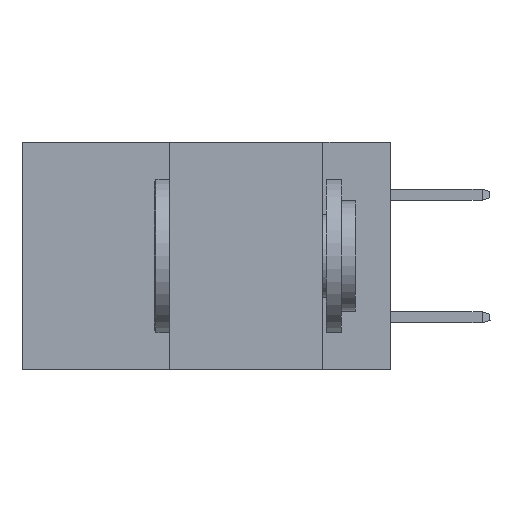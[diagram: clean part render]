
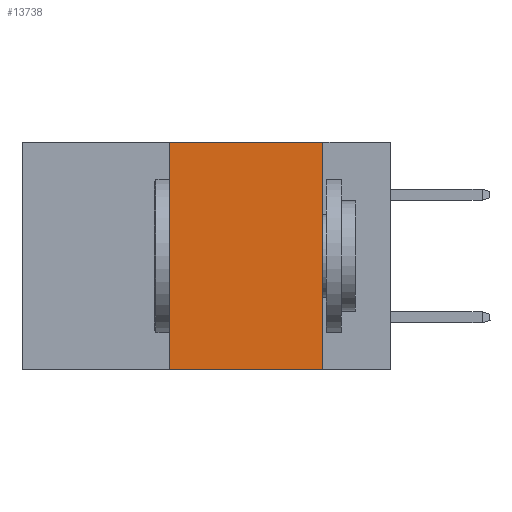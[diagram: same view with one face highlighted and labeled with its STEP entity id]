
A CAD part, left-side view. The second image highlights one B-rep face of the part: STEP entity #13738.
In plain terms, the highlighted planar face has unit normal (-1, 0, 0).
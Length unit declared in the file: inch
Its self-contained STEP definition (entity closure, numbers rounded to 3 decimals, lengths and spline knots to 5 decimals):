
#1080 = DIRECTION ( 'NONE',  ( 0., 0., 1. ) ) ;
#2075 = EDGE_CURVE ( 'NONE', #35773, #3460, #32425, .T. ) ;
#3299 = VERTEX_POINT ( 'NONE', #31021 ) ;
#3460 = VERTEX_POINT ( 'NONE', #13217 ) ;
#6713 = DIRECTION ( 'NONE',  ( 0., -1., 0. ) ) ;
#6886 = LINE ( 'NONE', #20181, #40118 ) ;
#6978 = VECTOR ( 'NONE', #37081, 39.37008 ) ;
#8865 = CARTESIAN_POINT ( 'NONE',  ( 0., 0.36, 0. ) ) ;
#10629 = VECTOR ( 'NONE', #36260, 39.37008 ) ;
#13023 = LINE ( 'NONE', #27232, #6978 ) ;
#13217 = CARTESIAN_POINT ( 'NONE',  ( 0., 0.11, -0.37 ) ) ;
#13467 = DIRECTION ( 'NONE',  ( 0., 0., -1. ) ) ;
#13738 = ADVANCED_FACE ( 'NONE', ( #32394 ), #39095, .F. ) ;
#18110 = EDGE_CURVE ( 'NONE', #3299, #3460, #38824, .T. ) ;
#18336 = VECTOR ( 'NONE', #6713, 39.37008 ) ;
#20181 = CARTESIAN_POINT ( 'NONE',  ( 0., 0.36, 0. ) ) ;
#21329 = ORIENTED_EDGE ( 'NONE', *, *, #34332, .F. ) ;
#26314 = ORIENTED_EDGE ( 'NONE', *, *, #2075, .T. ) ;
#26459 = DIRECTION ( 'NONE',  ( 1., 0., 0. ) ) ;
#26561 = CARTESIAN_POINT ( 'NONE',  ( 0., 0.11, 0. ) ) ;
#27232 = CARTESIAN_POINT ( 'NONE',  ( 0., 0.6, 0. ) ) ;
#28123 = ORIENTED_EDGE ( 'NONE', *, *, #36096, .F. ) ;
#29133 = EDGE_LOOP ( 'NONE', ( #31268, #21329, #28123, #26314 ) ) ;
#31021 = CARTESIAN_POINT ( 'NONE',  ( 0., 0.11, 0. ) ) ;
#31268 = ORIENTED_EDGE ( 'NONE', *, *, #18110, .F. ) ;
#31813 = CARTESIAN_POINT ( 'NONE',  ( 0., 0.6, -0.37 ) ) ;
#32303 = CARTESIAN_POINT ( 'NONE',  ( 0., 0.36, -0.37 ) ) ;
#32394 = FACE_OUTER_BOUND ( 'NONE', #29133, .T. ) ;
#32425 = LINE ( 'NONE', #31813, #18336 ) ;
#33072 = CARTESIAN_POINT ( 'NONE',  ( 0., 0.6, 0. ) ) ;
#34332 = EDGE_CURVE ( 'NONE', #38033, #3299, #13023, .T. ) ;
#35773 = VERTEX_POINT ( 'NONE', #32303 ) ;
#36096 = EDGE_CURVE ( 'NONE', #35773, #38033, #6886, .T. ) ;
#36260 = DIRECTION ( 'NONE',  ( 0., 0., -1. ) ) ;
#37081 = DIRECTION ( 'NONE',  ( 0., -1., 0. ) ) ;
#38033 = VERTEX_POINT ( 'NONE', #8865 ) ;
#38824 = LINE ( 'NONE', #26561, #10629 ) ;
#39095 = PLANE ( 'NONE',  #41014 ) ;
#40118 = VECTOR ( 'NONE', #1080, 39.37008 ) ;
#41014 = AXIS2_PLACEMENT_3D ( 'NONE', #33072, #26459, #13467 ) ;
